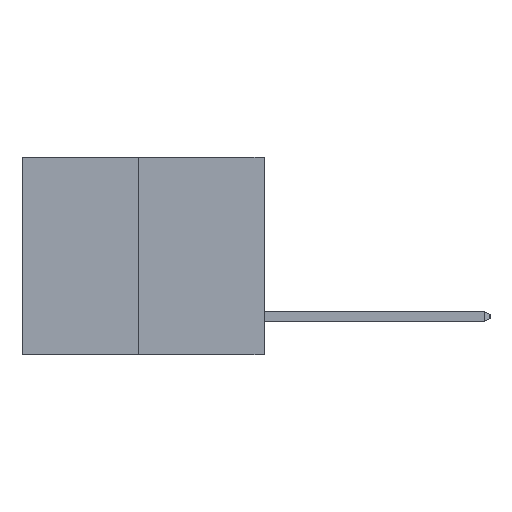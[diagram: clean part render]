
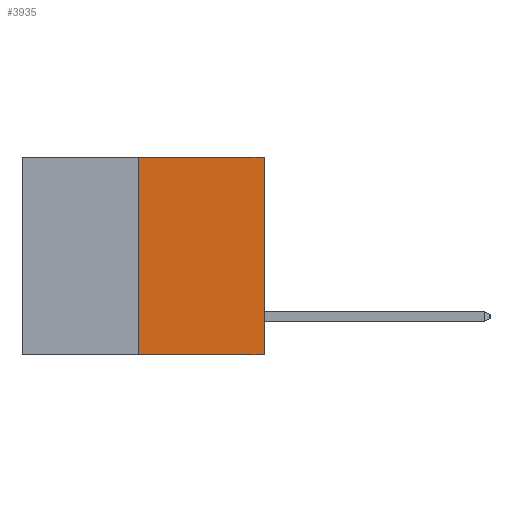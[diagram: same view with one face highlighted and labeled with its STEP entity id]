
A CAD part, left-side view. The second image highlights one B-rep face of the part: STEP entity #3935.
In plain terms, the highlighted planar face has unit normal (-1, 0, 0).
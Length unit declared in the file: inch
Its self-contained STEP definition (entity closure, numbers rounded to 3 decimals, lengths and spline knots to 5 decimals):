
#85 = ORIENTED_EDGE ( 'NONE', *, *, #6968, .F. ) ;
#521 = VECTOR ( 'NONE', #12287, 39.37008 ) ;
#917 = PLANE ( 'NONE',  #10593 ) ;
#1046 = CARTESIAN_POINT ( 'NONE',  ( 0., 0.6, 0. ) ) ;
#1626 = LINE ( 'NONE', #10060, #8981 ) ;
#2204 = VERTEX_POINT ( 'NONE', #7875 ) ;
#2532 = VECTOR ( 'NONE', #11121, 39.37008 ) ;
#2960 = EDGE_CURVE ( 'NONE', #8636, #2204, #1626, .T. ) ;
#3432 = CARTESIAN_POINT ( 'NONE',  ( 0., 0.312, -0.49 ) ) ;
#3935 = ADVANCED_FACE ( 'NONE', ( #12086 ), #917, .F. ) ;
#4149 = CARTESIAN_POINT ( 'NONE',  ( 0., 0.312, -0.49 ) ) ;
#4179 = CARTESIAN_POINT ( 'NONE',  ( 0., 0.312, 0. ) ) ;
#5137 = DIRECTION ( 'NONE',  ( 0., 0., 1. ) ) ;
#5531 = LINE ( 'NONE', #4149, #2532 ) ;
#6085 = LINE ( 'NONE', #8894, #8102 ) ;
#6809 = EDGE_LOOP ( 'NONE', ( #85, #7090, #12348, #8948 ) ) ;
#6968 = EDGE_CURVE ( 'NONE', #8636, #10480, #5531, .T. ) ;
#7090 = ORIENTED_EDGE ( 'NONE', *, *, #2960, .T. ) ;
#7457 = EDGE_CURVE ( 'NONE', #10480, #10656, #11447, .T. ) ;
#7875 = CARTESIAN_POINT ( 'NONE',  ( 0., 0., -0.49 ) ) ;
#7884 = DIRECTION ( 'NONE',  ( 1., 0., 0. ) ) ;
#8102 = VECTOR ( 'NONE', #5137, 39.37008 ) ;
#8636 = VERTEX_POINT ( 'NONE', #3432 ) ;
#8884 = DIRECTION ( 'NONE',  ( 0., 0., -1. ) ) ;
#8894 = CARTESIAN_POINT ( 'NONE',  ( 0., 0., 0. ) ) ;
#8948 = ORIENTED_EDGE ( 'NONE', *, *, #7457, .F. ) ;
#8981 = VECTOR ( 'NONE', #9204, 39.37008 ) ;
#9204 = DIRECTION ( 'NONE',  ( 0., -1., 0. ) ) ;
#9985 = EDGE_CURVE ( 'NONE', #2204, #10656, #6085, .T. ) ;
#10060 = CARTESIAN_POINT ( 'NONE',  ( 0., 0.6, -0.49 ) ) ;
#10480 = VERTEX_POINT ( 'NONE', #4179 ) ;
#10593 = AXIS2_PLACEMENT_3D ( 'NONE', #1046, #7884, #8884 ) ;
#10656 = VERTEX_POINT ( 'NONE', #11858 ) ;
#11121 = DIRECTION ( 'NONE',  ( 0., 0., 1. ) ) ;
#11329 = CARTESIAN_POINT ( 'NONE',  ( 0., 0.6, 0. ) ) ;
#11447 = LINE ( 'NONE', #11329, #521 ) ;
#11858 = CARTESIAN_POINT ( 'NONE',  ( 0., 0., 0. ) ) ;
#12086 = FACE_OUTER_BOUND ( 'NONE', #6809, .T. ) ;
#12287 = DIRECTION ( 'NONE',  ( 0., -1., 0. ) ) ;
#12348 = ORIENTED_EDGE ( 'NONE', *, *, #9985, .T. ) ;
